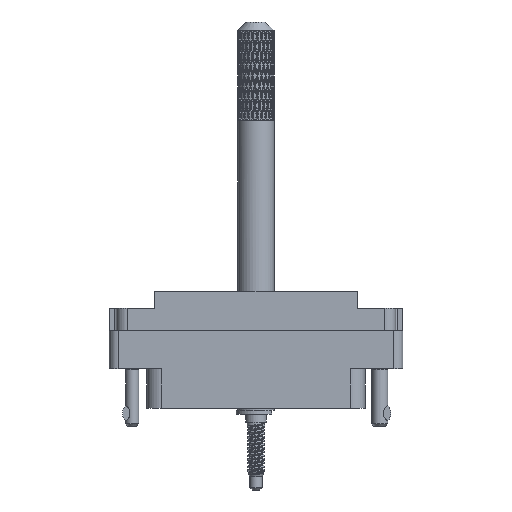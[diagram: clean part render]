
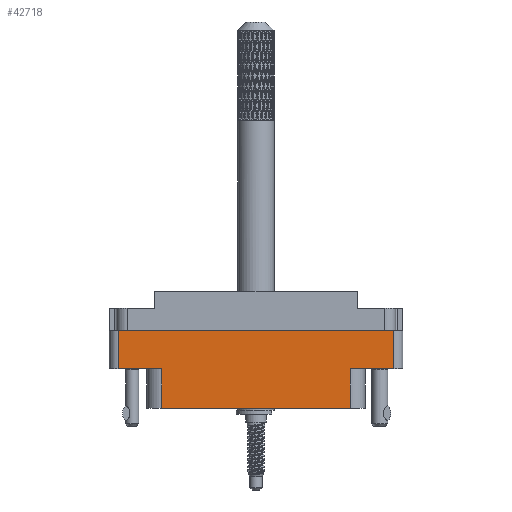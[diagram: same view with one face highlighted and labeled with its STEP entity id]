
A CAD part, front view. The second image highlights one B-rep face of the part: STEP entity #42718.
In plain terms, the highlighted planar face has unit normal (0, -1, 0).
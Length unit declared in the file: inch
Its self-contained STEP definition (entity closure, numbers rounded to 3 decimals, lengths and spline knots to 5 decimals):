
#5358 = CARTESIAN_POINT ( 'NONE',  ( -0.644, -0.438, -0.529 ) ) ;
#7218 = EDGE_CURVE ( 'NONE', #17087, #25657, #17394, .T. ) ;
#9536 = ORIENTED_EDGE ( 'NONE', *, *, #92575, .F. ) ;
#9552 = CARTESIAN_POINT ( 'NONE',  ( 0., -0.438, -0.529 ) ) ;
#12662 = DIRECTION ( 'NONE',  ( 0., 0., 1. ) ) ;
#14038 = VECTOR ( 'NONE', #28862, 39.37008 ) ;
#14344 = EDGE_CURVE ( 'NONE', #17087, #65985, #38069, .T. ) ;
#16021 = VECTOR ( 'NONE', #12662, 39.37008 ) ;
#16285 = FACE_OUTER_BOUND ( 'NONE', #54268, .T. ) ;
#17047 = DIRECTION ( 'NONE',  ( 0., 0., -1. ) ) ;
#17087 = VERTEX_POINT ( 'NONE', #73390 ) ;
#17394 = LINE ( 'NONE', #70737, #81110 ) ;
#17427 = ORIENTED_EDGE ( 'NONE', *, *, #74606, .T. ) ;
#19851 = VERTEX_POINT ( 'NONE', #35600 ) ;
#20332 = LINE ( 'NONE', #27300, #56764 ) ;
#25657 = VERTEX_POINT ( 'NONE', #29345 ) ;
#27300 = CARTESIAN_POINT ( 'NONE',  ( -0.938, -0.438, -0.798 ) ) ;
#28359 = ORIENTED_EDGE ( 'NONE', *, *, #7218, .F. ) ;
#28862 = DIRECTION ( 'NONE',  ( 0., 0., -1. ) ) ;
#29345 = CARTESIAN_POINT ( 'NONE',  ( 0.644, -0.438, -0.529 ) ) ;
#31487 = CARTESIAN_POINT ( 'NONE',  ( -0.938, -0.438, -0.529 ) ) ;
#34422 = ORIENTED_EDGE ( 'NONE', *, *, #54056, .F. ) ;
#35558 = LINE ( 'NONE', #67724, #36785 ) ;
#35600 = CARTESIAN_POINT ( 'NONE',  ( -0.644, -0.438, -0.529 ) ) ;
#36785 = VECTOR ( 'NONE', #85189, 39.37008 ) ;
#37384 = LINE ( 'NONE', #40570, #41268 ) ;
#37913 = PLANE ( 'NONE',  #92821 ) ;
#38069 = LINE ( 'NONE', #45669, #16021 ) ;
#38790 = CARTESIAN_POINT ( 'NONE',  ( 0.938, -0.438, -0.268 ) ) ;
#40570 = CARTESIAN_POINT ( 'NONE',  ( -0.938, -0.438, -0.798 ) ) ;
#40938 = DIRECTION ( 'NONE',  ( 1., 0., 0. ) ) ;
#41268 = VECTOR ( 'NONE', #40938, 39.37008 ) ;
#42718 = ADVANCED_FACE ( 'NONE', ( #16285 ), #37913, .T. ) ;
#43619 = VERTEX_POINT ( 'NONE', #63147 ) ;
#45669 = CARTESIAN_POINT ( 'NONE',  ( 0.938, -0.438, -0.798 ) ) ;
#46041 = DIRECTION ( 'NONE',  ( -1., 0., 0. ) ) ;
#46306 = DIRECTION ( 'NONE',  ( 0., 0., -1. ) ) ;
#48860 = ORIENTED_EDGE ( 'NONE', *, *, #76031, .T. ) ;
#54056 = EDGE_CURVE ( 'NONE', #25657, #91780, #64173, .T. ) ;
#54268 = EDGE_LOOP ( 'NONE', ( #48860, #59724, #34422, #28359, #99654, #74696, #9536, #17427 ) ) ;
#56764 = VECTOR ( 'NONE', #93881, 39.37008 ) ;
#59724 = ORIENTED_EDGE ( 'NONE', *, *, #64805, .T. ) ;
#60771 = LINE ( 'NONE', #5358, #14038 ) ;
#61506 = VECTOR ( 'NONE', #17047, 39.37008 ) ;
#63147 = CARTESIAN_POINT ( 'NONE',  ( -0.644, -0.438, -0.798 ) ) ;
#64173 = LINE ( 'NONE', #75175, #61506 ) ;
#64805 = EDGE_CURVE ( 'NONE', #43619, #91780, #37384, .T. ) ;
#65985 = VERTEX_POINT ( 'NONE', #38790 ) ;
#66252 = VECTOR ( 'NONE', #85088, 39.37008 ) ;
#67724 = CARTESIAN_POINT ( 'NONE',  ( -1., -0.438, -0.268 ) ) ;
#70737 = CARTESIAN_POINT ( 'NONE',  ( 0., -0.438, -0.529 ) ) ;
#73390 = CARTESIAN_POINT ( 'NONE',  ( 0.938, -0.438, -0.529 ) ) ;
#74606 = EDGE_CURVE ( 'NONE', #75060, #19851, #106517, .T. ) ;
#74696 = ORIENTED_EDGE ( 'NONE', *, *, #90390, .F. ) ;
#75060 = VERTEX_POINT ( 'NONE', #31487 ) ;
#75175 = CARTESIAN_POINT ( 'NONE',  ( 0.644, -0.438, -0.529 ) ) ;
#76031 = EDGE_CURVE ( 'NONE', #19851, #43619, #60771, .T. ) ;
#78654 = CARTESIAN_POINT ( 'NONE',  ( -0.938, -0.438, -0.798 ) ) ;
#81110 = VECTOR ( 'NONE', #46041, 39.37008 ) ;
#81238 = VERTEX_POINT ( 'NONE', #88629 ) ;
#85088 = DIRECTION ( 'NONE',  ( 1., 0., 0. ) ) ;
#85189 = DIRECTION ( 'NONE',  ( 1., 0., 0. ) ) ;
#88629 = CARTESIAN_POINT ( 'NONE',  ( -0.938, -0.438, -0.268 ) ) ;
#90390 = EDGE_CURVE ( 'NONE', #81238, #65985, #35558, .T. ) ;
#91780 = VERTEX_POINT ( 'NONE', #104430 ) ;
#92575 = EDGE_CURVE ( 'NONE', #75060, #81238, #20332, .T. ) ;
#92821 = AXIS2_PLACEMENT_3D ( 'NONE', #78654, #96109, #46306 ) ;
#93881 = DIRECTION ( 'NONE',  ( 0., 0., 1. ) ) ;
#96109 = DIRECTION ( 'NONE',  ( 0., -1., 0. ) ) ;
#99654 = ORIENTED_EDGE ( 'NONE', *, *, #14344, .T. ) ;
#104430 = CARTESIAN_POINT ( 'NONE',  ( 0.644, -0.438, -0.798 ) ) ;
#106517 = LINE ( 'NONE', #9552, #66252 ) ;
